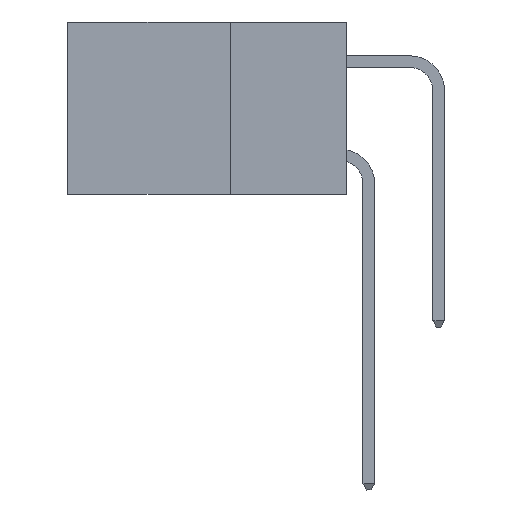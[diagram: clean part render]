
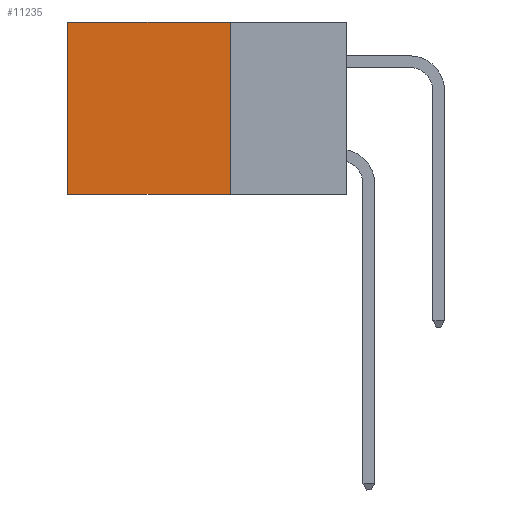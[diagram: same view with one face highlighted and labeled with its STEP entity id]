
A CAD part, left-side view. The second image highlights one B-rep face of the part: STEP entity #11235.
In plain terms, the highlighted planar face has unit normal (-1, 0, 0).
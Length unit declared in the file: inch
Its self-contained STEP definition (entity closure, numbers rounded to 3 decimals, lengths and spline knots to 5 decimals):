
#73 = VERTEX_POINT ( 'NONE', #3245 ) ;
#662 = AXIS2_PLACEMENT_3D ( 'NONE', #7647, #8332, #12044 ) ;
#728 = EDGE_LOOP ( 'NONE', ( #5407, #5421, #2528, #4542 ) ) ;
#1406 = PLANE ( 'NONE',  #662 ) ;
#1667 = VECTOR ( 'NONE', #3758, 39.37008 ) ;
#1800 = CARTESIAN_POINT ( 'NONE',  ( 0.2875, 0.6, 0. ) ) ;
#1822 = FACE_OUTER_BOUND ( 'NONE', #728, .T. ) ;
#2298 = VECTOR ( 'NONE', #8807, 39.37008 ) ;
#2391 = CARTESIAN_POINT ( 'NONE',  ( 0.2875, 0.25, -0.37 ) ) ;
#2528 = ORIENTED_EDGE ( 'NONE', *, *, #10871, .F. ) ;
#3165 = EDGE_CURVE ( 'NONE', #73, #4977, #8805, .T. ) ;
#3245 = CARTESIAN_POINT ( 'NONE',  ( 0.2875, 0.25, 0. ) ) ;
#3758 = DIRECTION ( 'NONE',  ( 0., 0., -1. ) ) ;
#3805 = LINE ( 'NONE', #10421, #1667 ) ;
#4462 = VECTOR ( 'NONE', #11985, 39.37008 ) ;
#4499 = VERTEX_POINT ( 'NONE', #7578 ) ;
#4542 = ORIENTED_EDGE ( 'NONE', *, *, #3165, .T. ) ;
#4909 = LINE ( 'NONE', #8444, #10514 ) ;
#4977 = VERTEX_POINT ( 'NONE', #1800 ) ;
#5407 = ORIENTED_EDGE ( 'NONE', *, *, #8563, .T. ) ;
#5421 = ORIENTED_EDGE ( 'NONE', *, *, #7847, .F. ) ;
#6335 = VERTEX_POINT ( 'NONE', #9580 ) ;
#7578 = CARTESIAN_POINT ( 'NONE',  ( 0.2875, 0.25, -0.37 ) ) ;
#7647 = CARTESIAN_POINT ( 'NONE',  ( 0.2875, 0.25, 0. ) ) ;
#7847 = EDGE_CURVE ( 'NONE', #4499, #6335, #11424, .T. ) ;
#8332 = DIRECTION ( 'NONE',  ( 1., 0., 0. ) ) ;
#8361 = DIRECTION ( 'NONE',  ( 0., 0., -1. ) ) ;
#8444 = CARTESIAN_POINT ( 'NONE',  ( 0.2875, 0.6, 0. ) ) ;
#8563 = EDGE_CURVE ( 'NONE', #4977, #6335, #4909, .T. ) ;
#8805 = LINE ( 'NONE', #9744, #2298 ) ;
#8807 = DIRECTION ( 'NONE',  ( 0., 1., 0. ) ) ;
#9580 = CARTESIAN_POINT ( 'NONE',  ( 0.2875, 0.6, -0.37 ) ) ;
#9744 = CARTESIAN_POINT ( 'NONE',  ( 0.2875, 0.25, 0. ) ) ;
#10421 = CARTESIAN_POINT ( 'NONE',  ( 0.2875, 0.25, 0. ) ) ;
#10514 = VECTOR ( 'NONE', #8361, 39.37008 ) ;
#10871 = EDGE_CURVE ( 'NONE', #73, #4499, #3805, .T. ) ;
#11235 = ADVANCED_FACE ( 'NONE', ( #1822 ), #1406, .F. ) ;
#11424 = LINE ( 'NONE', #2391, #4462 ) ;
#11985 = DIRECTION ( 'NONE',  ( 0., 1., 0. ) ) ;
#12044 = DIRECTION ( 'NONE',  ( 0., 0., -1. ) ) ;
